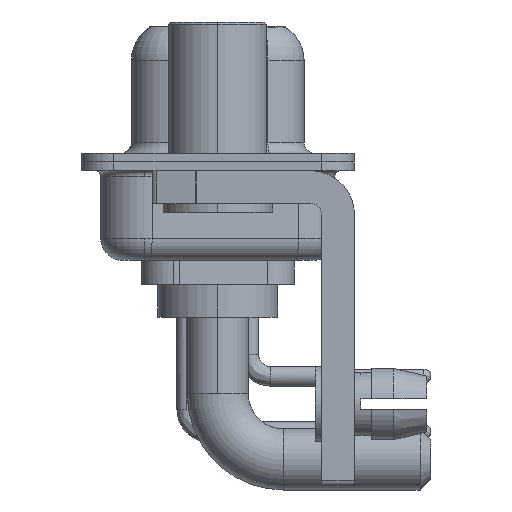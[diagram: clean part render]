
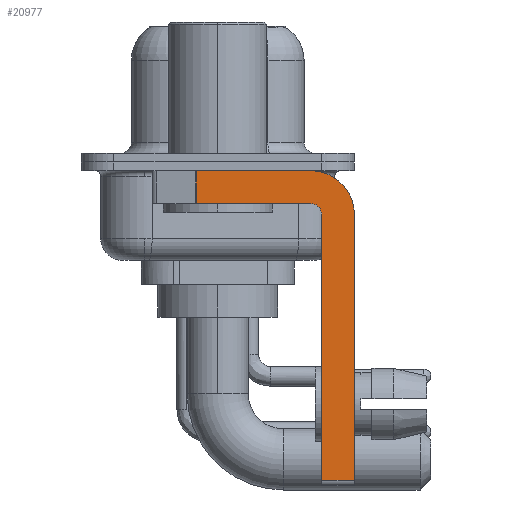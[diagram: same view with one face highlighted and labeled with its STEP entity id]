
A CAD part, left-side view. The second image highlights one B-rep face of the part: STEP entity #20977.
In plain terms, the highlighted planar face has unit normal (-1, 0, 0).
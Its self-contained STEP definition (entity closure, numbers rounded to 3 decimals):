
#505 = LINE ( 'NONE', #11143, #3932 ) ;
#766 = ORIENTED_EDGE ( 'NONE', *, *, #15896, .F. ) ;
#915 = EDGE_CURVE ( 'NONE', #7346, #5583, #26179, .T. ) ;
#1626 = VECTOR ( 'NONE', #4660, 1000. ) ;
#2056 = CARTESIAN_POINT ( 'NONE',  ( -2.9, -4.25, -0.4 ) ) ;
#2931 = ORIENTED_EDGE ( 'NONE', *, *, #17400, .F. ) ;
#2953 = DIRECTION ( 'NONE',  ( 0., 1., 0. ) ) ;
#3932 = VECTOR ( 'NONE', #26409, 1000. ) ;
#4100 = CARTESIAN_POINT ( 'NONE',  ( -2.9, -4.25, -1.9 ) ) ;
#4660 = DIRECTION ( 'NONE',  ( 0., 0., 1. ) ) ;
#5534 = LINE ( 'NONE', #12070, #22049 ) ;
#5583 = VERTEX_POINT ( 'NONE', #5860 ) ;
#5678 = EDGE_CURVE ( 'NONE', #22476, #23144, #14825, .T. ) ;
#5860 = CARTESIAN_POINT ( 'NONE',  ( -2.9, -4.75, -2.4 ) ) ;
#6073 = VERTEX_POINT ( 'NONE', #6370 ) ;
#6190 = DIRECTION ( 'NONE',  ( 0., 0., -1. ) ) ;
#6370 = CARTESIAN_POINT ( 'NONE',  ( -2.9, 0.978, -1.9 ) ) ;
#6402 = DIRECTION ( 'NONE',  ( 1., 0., 0. ) ) ;
#6590 = AXIS2_PLACEMENT_3D ( 'NONE', #21316, #12963, #21597 ) ;
#7346 = VERTEX_POINT ( 'NONE', #15585 ) ;
#7417 = ORIENTED_EDGE ( 'NONE', *, *, #8557, .F. ) ;
#8317 = CARTESIAN_POINT ( 'NONE',  ( -2.9, -4.25, -2.4 ) ) ;
#8557 = EDGE_CURVE ( 'NONE', #23144, #18514, #27606, .T. ) ;
#8676 = DIRECTION ( 'NONE',  ( 0., 0., -1. ) ) ;
#10439 = EDGE_CURVE ( 'NONE', #7346, #18514, #12043, .T. ) ;
#11143 = CARTESIAN_POINT ( 'NONE',  ( -2.9, 3., -0.4 ) ) ;
#12043 = LINE ( 'NONE', #20678, #26354 ) ;
#12070 = CARTESIAN_POINT ( 'NONE',  ( -2.9, 0.978, -1.9 ) ) ;
#12645 = CARTESIAN_POINT ( 'NONE',  ( -2.9, -4.25, -1.9 ) ) ;
#12963 = DIRECTION ( 'NONE',  ( -1., 0., 0. ) ) ;
#13159 = DIRECTION ( 'NONE',  ( 0., -1., 0. ) ) ;
#13347 = CARTESIAN_POINT ( 'NONE',  ( -2.9, -6.25, -2.4 ) ) ;
#14455 = CARTESIAN_POINT ( 'NONE',  ( -2.9, 0.978, -0.4 ) ) ;
#14825 = CIRCLE ( 'NONE', #24900, 2. ) ;
#15019 = VECTOR ( 'NONE', #2953, 1000. ) ;
#15119 = FACE_OUTER_BOUND ( 'NONE', #26911, .T. ) ;
#15345 = CARTESIAN_POINT ( 'NONE',  ( -2.9, -4.25, -2.4 ) ) ;
#15442 = CARTESIAN_POINT ( 'NONE',  ( -2.9, -4.75, -14.8 ) ) ;
#15585 = CARTESIAN_POINT ( 'NONE',  ( -2.9, -4.75, -14.55 ) ) ;
#15896 = EDGE_CURVE ( 'NONE', #19090, #22476, #505, .T. ) ;
#16737 = DIRECTION ( 'NONE',  ( 0., 0., -1. ) ) ;
#17238 = PLANE ( 'NONE',  #25511 ) ;
#17400 = EDGE_CURVE ( 'NONE', #22974, #6073, #23499, .T. ) ;
#17444 = CIRCLE ( 'NONE', #6590, 0.5 ) ;
#18428 = DIRECTION ( 'NONE',  ( 0., 0., -1. ) ) ;
#18514 = VERTEX_POINT ( 'NONE', #26939 ) ;
#18555 = ORIENTED_EDGE ( 'NONE', *, *, #10439, .T. ) ;
#19090 = VERTEX_POINT ( 'NONE', #14455 ) ;
#20678 = CARTESIAN_POINT ( 'NONE',  ( -2.9, -4.25, -14.55 ) ) ;
#20977 = ADVANCED_FACE ( 'NONE', ( #15119 ), #17238, .F. ) ;
#21303 = VECTOR ( 'NONE', #16737, 1000. ) ;
#21316 = CARTESIAN_POINT ( 'NONE',  ( -2.9, -4.25, -2.4 ) ) ;
#21597 = DIRECTION ( 'NONE',  ( 0., 0., 1. ) ) ;
#22049 = VECTOR ( 'NONE', #18428, 1000. ) ;
#22476 = VERTEX_POINT ( 'NONE', #2056 ) ;
#22560 = EDGE_CURVE ( 'NONE', #5583, #22974, #17444, .T. ) ;
#22974 = VERTEX_POINT ( 'NONE', #12645 ) ;
#23144 = VERTEX_POINT ( 'NONE', #13347 ) ;
#23475 = DIRECTION ( 'NONE',  ( 1., 0., 0. ) ) ;
#23499 = LINE ( 'NONE', #4100, #15019 ) ;
#24653 = ORIENTED_EDGE ( 'NONE', *, *, #915, .F. ) ;
#24900 = AXIS2_PLACEMENT_3D ( 'NONE', #15345, #6402, #8676 ) ;
#24950 = EDGE_CURVE ( 'NONE', #19090, #6073, #5534, .T. ) ;
#25511 = AXIS2_PLACEMENT_3D ( 'NONE', #8317, #23475, #6190 ) ;
#26179 = LINE ( 'NONE', #15442, #1626 ) ;
#26354 = VECTOR ( 'NONE', #13159, 1000. ) ;
#26409 = DIRECTION ( 'NONE',  ( 0., -1., 0. ) ) ;
#26893 = ORIENTED_EDGE ( 'NONE', *, *, #22560, .F. ) ;
#26911 = EDGE_LOOP ( 'NONE', ( #766, #27746, #2931, #26893, #24653, #18555, #7417, #27777 ) ) ;
#26939 = CARTESIAN_POINT ( 'NONE',  ( -2.9, -6.25, -14.55 ) ) ;
#27468 = CARTESIAN_POINT ( 'NONE',  ( -2.9, -6.25, -2.4 ) ) ;
#27606 = LINE ( 'NONE', #27468, #21303 ) ;
#27746 = ORIENTED_EDGE ( 'NONE', *, *, #24950, .T. ) ;
#27777 = ORIENTED_EDGE ( 'NONE', *, *, #5678, .F. ) ;
